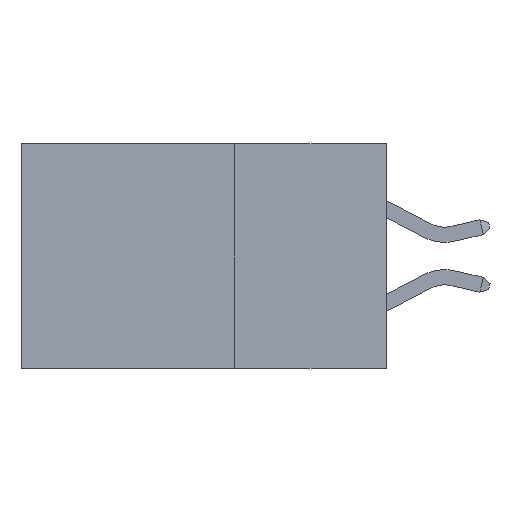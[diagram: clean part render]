
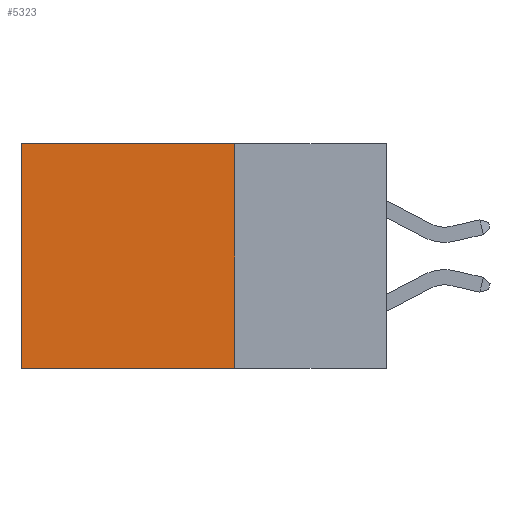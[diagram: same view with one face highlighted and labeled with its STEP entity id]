
A CAD part, left-side view. The second image highlights one B-rep face of the part: STEP entity #5323.
In plain terms, the highlighted planar face has unit normal (-1, 0, 0).
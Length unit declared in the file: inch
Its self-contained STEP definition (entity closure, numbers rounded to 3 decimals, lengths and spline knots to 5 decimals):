
#200 = DIRECTION ( 'NONE',  ( 0., 0., -1. ) ) ;
#272 = VERTEX_POINT ( 'NONE', #893 ) ;
#442 = ORIENTED_EDGE ( 'NONE', *, *, #3353, .T. ) ;
#893 = CARTESIAN_POINT ( 'NONE',  ( 0.2615, 0.25, 0. ) ) ;
#901 = DIRECTION ( 'NONE',  ( 0., 0., -1. ) ) ;
#905 = VERTEX_POINT ( 'NONE', #5674 ) ;
#907 = CARTESIAN_POINT ( 'NONE',  ( 0.2615, 0.25, -0.37 ) ) ;
#1179 = ORIENTED_EDGE ( 'NONE', *, *, #3308, .T. ) ;
#1551 = EDGE_CURVE ( 'NONE', #272, #905, #6831, .T. ) ;
#1664 = CARTESIAN_POINT ( 'NONE',  ( 0.2615, 0.6, -0.37 ) ) ;
#1766 = DIRECTION ( 'NONE',  ( 0., 1., 0. ) ) ;
#1793 = DIRECTION ( 'NONE',  ( 1., 0., 0. ) ) ;
#1920 = VECTOR ( 'NONE', #9731, 39.37008 ) ;
#2485 = DIRECTION ( 'NONE',  ( 0., 0., -1. ) ) ;
#2983 = VECTOR ( 'NONE', #901, 39.37008 ) ;
#3210 = CARTESIAN_POINT ( 'NONE',  ( 0.2615, 0.6, -0.37 ) ) ;
#3308 = EDGE_CURVE ( 'NONE', #272, #8967, #10274, .T. ) ;
#3353 = EDGE_CURVE ( 'NONE', #8967, #9792, #6193, .T. ) ;
#3660 = LINE ( 'NONE', #6526, #1920 ) ;
#4325 = EDGE_CURVE ( 'NONE', #905, #9792, #3660, .T. ) ;
#4893 = FACE_OUTER_BOUND ( 'NONE', #5995, .T. ) ;
#4899 = PLANE ( 'NONE',  #6592 ) ;
#5251 = ORIENTED_EDGE ( 'NONE', *, *, #4325, .F. ) ;
#5323 = ADVANCED_FACE ( 'NONE', ( #4893 ), #4899, .F. ) ;
#5674 = CARTESIAN_POINT ( 'NONE',  ( 0.2615, 0.25, -0.37 ) ) ;
#5683 = CARTESIAN_POINT ( 'NONE',  ( 0.2615, 0.25, -0.37 ) ) ;
#5700 = VECTOR ( 'NONE', #2485, 39.37008 ) ;
#5995 = EDGE_LOOP ( 'NONE', ( #442, #5251, #8156, #1179 ) ) ;
#6193 = LINE ( 'NONE', #1664, #5700 ) ;
#6526 = CARTESIAN_POINT ( 'NONE',  ( 0.2615, 0.25, -0.37 ) ) ;
#6538 = CARTESIAN_POINT ( 'NONE',  ( 0.2615, 0.25, 0. ) ) ;
#6592 = AXIS2_PLACEMENT_3D ( 'NONE', #907, #1793, #200 ) ;
#6831 = LINE ( 'NONE', #5683, #2983 ) ;
#8156 = ORIENTED_EDGE ( 'NONE', *, *, #1551, .F. ) ;
#8191 = VECTOR ( 'NONE', #1766, 39.37008 ) ;
#8209 = CARTESIAN_POINT ( 'NONE',  ( 0.2615, 0.6, 0. ) ) ;
#8967 = VERTEX_POINT ( 'NONE', #8209 ) ;
#9731 = DIRECTION ( 'NONE',  ( 0., 1., 0. ) ) ;
#9792 = VERTEX_POINT ( 'NONE', #3210 ) ;
#10274 = LINE ( 'NONE', #6538, #8191 ) ;
